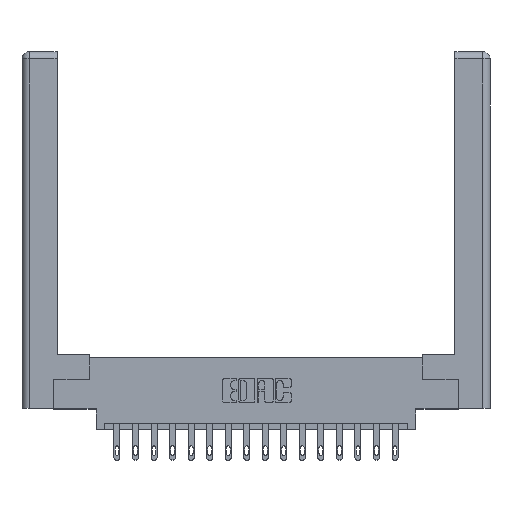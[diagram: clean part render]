
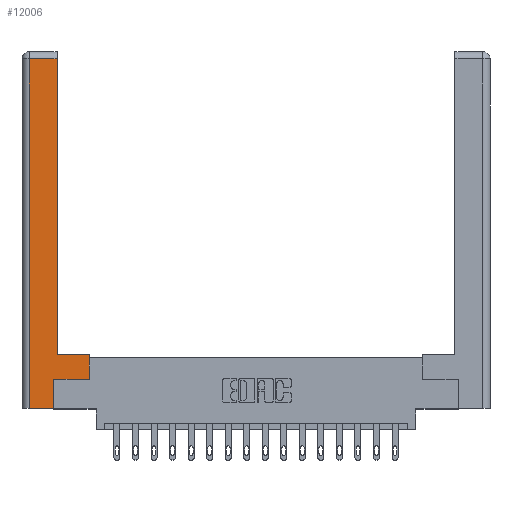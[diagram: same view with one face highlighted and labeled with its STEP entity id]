
A CAD part, top view. The second image highlights one B-rep face of the part: STEP entity #12006.
In plain terms, the highlighted planar face has unit normal (0, 0, 1).
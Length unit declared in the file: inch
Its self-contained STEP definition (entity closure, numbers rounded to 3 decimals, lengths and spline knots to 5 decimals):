
#34 = LINE ( 'NONE', #1484, #16136 ) ;
#357 = CARTESIAN_POINT ( 'NONE',  ( 0.0615, 2.94, 0. ) ) ;
#464 = CARTESIAN_POINT ( 'NONE',  ( 0.265, 0., 0. ) ) ;
#1007 = DIRECTION ( 'NONE',  ( 0., -1., 0. ) ) ;
#1114 = VERTEX_POINT ( 'NONE', #1949 ) ;
#1282 = DIRECTION ( 'NONE',  ( -1., 0., 0. ) ) ;
#1473 = VECTOR ( 'NONE', #2982, 39.37008 ) ;
#1484 = CARTESIAN_POINT ( 'NONE',  ( 0.265, 0., 0. ) ) ;
#1642 = LINE ( 'NONE', #14729, #16606 ) ;
#1830 = EDGE_CURVE ( 'NONE', #2454, #14261, #2506, .T. ) ;
#1949 = CARTESIAN_POINT ( 'NONE',  ( 0.295, 0.45, 0. ) ) ;
#2299 = EDGE_CURVE ( 'NONE', #1114, #16762, #6235, .T. ) ;
#2454 = VERTEX_POINT ( 'NONE', #464 ) ;
#2506 = LINE ( 'NONE', #10713, #6465 ) ;
#2731 = EDGE_CURVE ( 'NONE', #12144, #2454, #34, .T. ) ;
#2924 = LINE ( 'NONE', #7057, #15213 ) ;
#2982 = DIRECTION ( 'NONE',  ( -1., 0., 0. ) ) ;
#3182 = ORIENTED_EDGE ( 'NONE', *, *, #2299, .T. ) ;
#3473 = ORIENTED_EDGE ( 'NONE', *, *, #13822, .T. ) ;
#3605 = LINE ( 'NONE', #3999, #18355 ) ;
#3999 = CARTESIAN_POINT ( 'NONE',  ( 0.565, 0.45, 0. ) ) ;
#4184 = DIRECTION ( 'NONE',  ( -1., 0., 0. ) ) ;
#4947 = DIRECTION ( 'NONE',  ( 0., 1., 0. ) ) ;
#5412 = DIRECTION ( 'NONE',  ( 0., 1., 0. ) ) ;
#5729 = VERTEX_POINT ( 'NONE', #12522 ) ;
#6235 = LINE ( 'NONE', #16030, #12064 ) ;
#6465 = VECTOR ( 'NONE', #4947, 39.37008 ) ;
#6854 = EDGE_LOOP ( 'NONE', ( #3182, #3473, #10022, #11741, #8738, #8694, #11978, #17742 ) ) ;
#7045 = PLANE ( 'NONE',  #11914 ) ;
#7057 = CARTESIAN_POINT ( 'NONE',  ( 0.0615, 0., 0. ) ) ;
#7788 = CARTESIAN_POINT ( 'NONE',  ( 0.565, 0.245, 0. ) ) ;
#8157 = EDGE_CURVE ( 'NONE', #5729, #1114, #16638, .T. ) ;
#8391 = CARTESIAN_POINT ( 'NONE',  ( 0.295, 0.45, 0. ) ) ;
#8694 = ORIENTED_EDGE ( 'NONE', *, *, #15316, .T. ) ;
#8738 = ORIENTED_EDGE ( 'NONE', *, *, #1830, .T. ) ;
#8805 = CARTESIAN_POINT ( 'NONE',  ( 0.565, 0.245, 0. ) ) ;
#9035 = VERTEX_POINT ( 'NONE', #8805 ) ;
#9184 = DIRECTION ( 'NONE',  ( 1., 0., 0. ) ) ;
#9907 = DIRECTION ( 'NONE',  ( 0., 1., 0. ) ) ;
#9914 = EDGE_CURVE ( 'NONE', #11448, #12144, #2924, .T. ) ;
#10022 = ORIENTED_EDGE ( 'NONE', *, *, #9914, .T. ) ;
#10713 = CARTESIAN_POINT ( 'NONE',  ( 0.265, 0.245, 0. ) ) ;
#11448 = VERTEX_POINT ( 'NONE', #357 ) ;
#11741 = ORIENTED_EDGE ( 'NONE', *, *, #2731, .T. ) ;
#11914 = AXIS2_PLACEMENT_3D ( 'NONE', #17130, #17018, #4184 ) ;
#11978 = ORIENTED_EDGE ( 'NONE', *, *, #14589, .T. ) ;
#12006 = ADVANCED_FACE ( 'NONE', ( #16079 ), #7045, .F. ) ;
#12064 = VECTOR ( 'NONE', #9907, 39.37008 ) ;
#12144 = VERTEX_POINT ( 'NONE', #13479 ) ;
#12522 = CARTESIAN_POINT ( 'NONE',  ( 0.565, 0.45, 0. ) ) ;
#13479 = CARTESIAN_POINT ( 'NONE',  ( 0.0615, 0., 0. ) ) ;
#13822 = EDGE_CURVE ( 'NONE', #16762, #11448, #1642, .T. ) ;
#13919 = CARTESIAN_POINT ( 'NONE',  ( 0.265, 0.245, 0. ) ) ;
#14261 = VERTEX_POINT ( 'NONE', #13919 ) ;
#14589 = EDGE_CURVE ( 'NONE', #9035, #5729, #3605, .T. ) ;
#14729 = CARTESIAN_POINT ( 'NONE',  ( 0.0615, 2.94, 0. ) ) ;
#14760 = VECTOR ( 'NONE', #9184, 39.37008 ) ;
#15213 = VECTOR ( 'NONE', #1007, 39.37008 ) ;
#15316 = EDGE_CURVE ( 'NONE', #14261, #9035, #16557, .T. ) ;
#15838 = DIRECTION ( 'NONE',  ( 1., 0., 0. ) ) ;
#16030 = CARTESIAN_POINT ( 'NONE',  ( 0.295, 3., 0. ) ) ;
#16079 = FACE_OUTER_BOUND ( 'NONE', #6854, .T. ) ;
#16136 = VECTOR ( 'NONE', #15838, 39.37008 ) ;
#16169 = CARTESIAN_POINT ( 'NONE',  ( 0.295, 2.94, 0. ) ) ;
#16557 = LINE ( 'NONE', #7788, #14760 ) ;
#16606 = VECTOR ( 'NONE', #1282, 39.37008 ) ;
#16638 = LINE ( 'NONE', #8391, #1473 ) ;
#16762 = VERTEX_POINT ( 'NONE', #16169 ) ;
#17018 = DIRECTION ( 'NONE',  ( 0., 0., -1. ) ) ;
#17130 = CARTESIAN_POINT ( 'NONE',  ( 0., 0., 0. ) ) ;
#17742 = ORIENTED_EDGE ( 'NONE', *, *, #8157, .T. ) ;
#18355 = VECTOR ( 'NONE', #5412, 39.37008 ) ;
